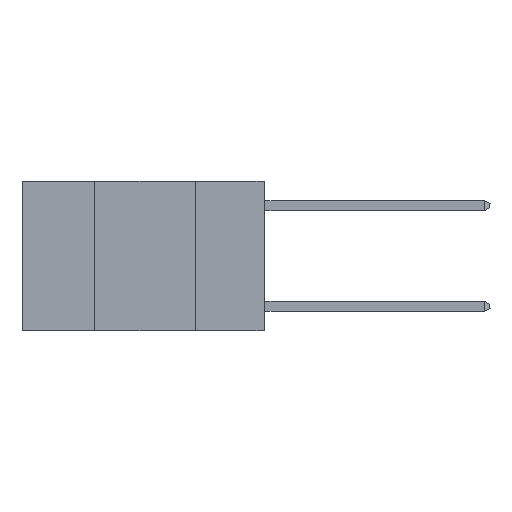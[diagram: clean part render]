
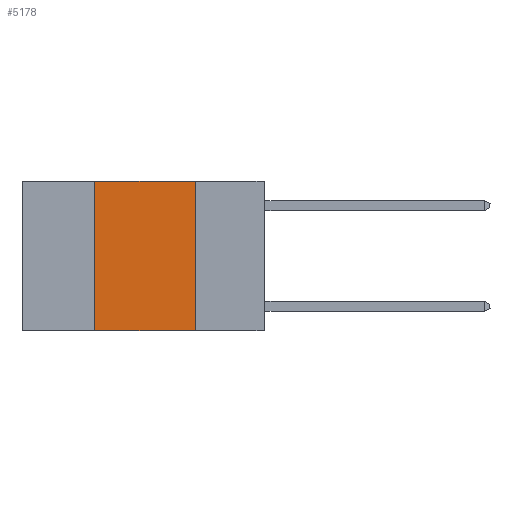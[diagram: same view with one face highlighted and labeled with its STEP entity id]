
A CAD part, left-side view. The second image highlights one B-rep face of the part: STEP entity #5178.
In plain terms, the highlighted planar face has unit normal (-1, 0, 0).
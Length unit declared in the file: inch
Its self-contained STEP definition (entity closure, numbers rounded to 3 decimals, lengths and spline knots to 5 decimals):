
#784 = EDGE_CURVE ( 'NONE', #14102, #21188, #24221, .T. ) ;
#1921 = VERTEX_POINT ( 'NONE', #2343 ) ;
#2343 = CARTESIAN_POINT ( 'NONE',  ( 0., 0.17, -0.37 ) ) ;
#3410 = EDGE_LOOP ( 'NONE', ( #20374, #9273, #23492, #20022 ) ) ;
#4146 = LINE ( 'NONE', #22775, #11634 ) ;
#5178 = ADVANCED_FACE ( 'NONE', ( #20511 ), #18640, .F. ) ;
#5756 = DIRECTION ( 'NONE',  ( 0., -1., 0. ) ) ;
#5880 = DIRECTION ( 'NONE',  ( 0., 0., 1. ) ) ;
#6022 = CARTESIAN_POINT ( 'NONE',  ( 0., 0.17, 0. ) ) ;
#6176 = VECTOR ( 'NONE', #8456, 39.37008 ) ;
#7345 = CARTESIAN_POINT ( 'NONE',  ( 0., 0.6, 0. ) ) ;
#7940 = CARTESIAN_POINT ( 'NONE',  ( 0., 0.42, -0.37 ) ) ;
#8456 = DIRECTION ( 'NONE',  ( 0., 0., -1. ) ) ;
#9273 = ORIENTED_EDGE ( 'NONE', *, *, #784, .F. ) ;
#10075 = LINE ( 'NONE', #10308, #6176 ) ;
#10308 = CARTESIAN_POINT ( 'NONE',  ( 0., 0.17, 0. ) ) ;
#10582 = CARTESIAN_POINT ( 'NONE',  ( 0., 0.42, 0. ) ) ;
#11279 = VECTOR ( 'NONE', #22398, 39.37008 ) ;
#11634 = VECTOR ( 'NONE', #5880, 39.37008 ) ;
#12090 = EDGE_CURVE ( 'NONE', #21188, #1921, #10075, .T. ) ;
#12934 = EDGE_CURVE ( 'NONE', #22980, #14102, #4146, .T. ) ;
#14102 = VERTEX_POINT ( 'NONE', #10582 ) ;
#14576 = VECTOR ( 'NONE', #5756, 39.37008 ) ;
#15137 = CARTESIAN_POINT ( 'NONE',  ( 0., 0.6, -0.37 ) ) ;
#16599 = DIRECTION ( 'NONE',  ( 1., 0., 0. ) ) ;
#18640 = PLANE ( 'NONE',  #18656 ) ;
#18656 = AXIS2_PLACEMENT_3D ( 'NONE', #20154, #16599, #22248 ) ;
#19216 = EDGE_CURVE ( 'NONE', #22980, #1921, #23022, .T. ) ;
#20022 = ORIENTED_EDGE ( 'NONE', *, *, #19216, .T. ) ;
#20154 = CARTESIAN_POINT ( 'NONE',  ( 0., 0.6, 0. ) ) ;
#20374 = ORIENTED_EDGE ( 'NONE', *, *, #12090, .F. ) ;
#20511 = FACE_OUTER_BOUND ( 'NONE', #3410, .T. ) ;
#21188 = VERTEX_POINT ( 'NONE', #6022 ) ;
#22248 = DIRECTION ( 'NONE',  ( 0., 0., -1. ) ) ;
#22398 = DIRECTION ( 'NONE',  ( 0., -1., 0. ) ) ;
#22775 = CARTESIAN_POINT ( 'NONE',  ( 0., 0.42, 0. ) ) ;
#22980 = VERTEX_POINT ( 'NONE', #7940 ) ;
#23022 = LINE ( 'NONE', #15137, #14576 ) ;
#23492 = ORIENTED_EDGE ( 'NONE', *, *, #12934, .F. ) ;
#24221 = LINE ( 'NONE', #7345, #11279 ) ;
